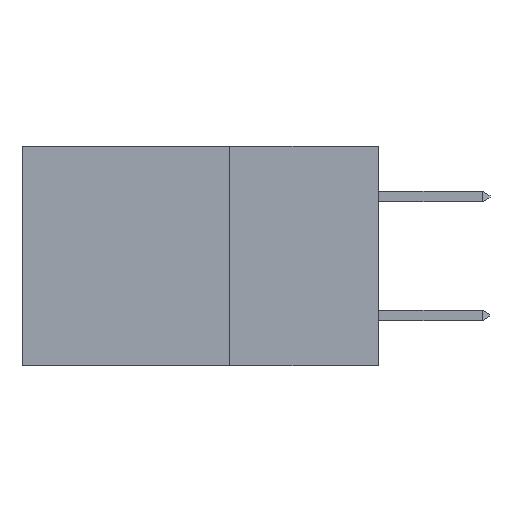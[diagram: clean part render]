
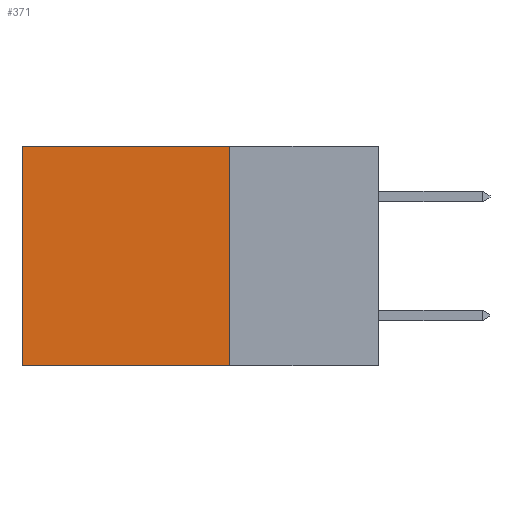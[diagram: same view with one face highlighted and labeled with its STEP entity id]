
A CAD part, left-side view. The second image highlights one B-rep face of the part: STEP entity #371.
In plain terms, the highlighted planar face has unit normal (-1, 0, 0).
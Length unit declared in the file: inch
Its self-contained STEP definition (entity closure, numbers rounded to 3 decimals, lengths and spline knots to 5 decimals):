
#371 = ADVANCED_FACE ( 'NONE', ( #16204 ), #21209, .F. ) ;
#437 = DIRECTION ( 'NONE',  ( 0., 0., -1. ) ) ;
#588 = LINE ( 'NONE', #5844, #9871 ) ;
#594 = DIRECTION ( 'NONE',  ( 1., 0., 0. ) ) ;
#700 = CARTESIAN_POINT ( 'NONE',  ( 0.298, 0.25, 0. ) ) ;
#2138 = CARTESIAN_POINT ( 'NONE',  ( 0.298, 0.25, 0. ) ) ;
#2840 = ORIENTED_EDGE ( 'NONE', *, *, #19943, .T. ) ;
#3973 = DIRECTION ( 'NONE',  ( 0., 1., 0. ) ) ;
#4459 = CARTESIAN_POINT ( 'NONE',  ( 0.298, 0.6, 0. ) ) ;
#4568 = LINE ( 'NONE', #14519, #19767 ) ;
#5844 = CARTESIAN_POINT ( 'NONE',  ( 0.298, 0.25, 0. ) ) ;
#6320 = VECTOR ( 'NONE', #3973, 39.37008 ) ;
#6471 = VERTEX_POINT ( 'NONE', #9774 ) ;
#6593 = CARTESIAN_POINT ( 'NONE',  ( 0.298, 0.6, -0.37 ) ) ;
#6660 = DIRECTION ( 'NONE',  ( 0., 0., -1. ) ) ;
#7316 = CARTESIAN_POINT ( 'NONE',  ( 0.298, 0.25, 0. ) ) ;
#7697 = DIRECTION ( 'NONE',  ( 0., 0., -1. ) ) ;
#8501 = EDGE_CURVE ( 'NONE', #21553, #23458, #11255, .T. ) ;
#8518 = EDGE_LOOP ( 'NONE', ( #2840, #14229, #15672, #9658 ) ) ;
#9658 = ORIENTED_EDGE ( 'NONE', *, *, #8501, .T. ) ;
#9774 = CARTESIAN_POINT ( 'NONE',  ( 0.298, 0.25, -0.37 ) ) ;
#9871 = VECTOR ( 'NONE', #7697, 39.37008 ) ;
#11255 = LINE ( 'NONE', #2138, #6320 ) ;
#13878 = VERTEX_POINT ( 'NONE', #6593 ) ;
#14229 = ORIENTED_EDGE ( 'NONE', *, *, #21485, .F. ) ;
#14519 = CARTESIAN_POINT ( 'NONE',  ( 0.298, 0.25, -0.37 ) ) ;
#15672 = ORIENTED_EDGE ( 'NONE', *, *, #20323, .F. ) ;
#16204 = FACE_OUTER_BOUND ( 'NONE', #8518, .T. ) ;
#17720 = CARTESIAN_POINT ( 'NONE',  ( 0.298, 0.6, 0. ) ) ;
#19767 = VECTOR ( 'NONE', #19860, 39.37008 ) ;
#19860 = DIRECTION ( 'NONE',  ( 0., 1., 0. ) ) ;
#19943 = EDGE_CURVE ( 'NONE', #23458, #13878, #22610, .T. ) ;
#20091 = AXIS2_PLACEMENT_3D ( 'NONE', #700, #594, #437 ) ;
#20323 = EDGE_CURVE ( 'NONE', #21553, #6471, #588, .T. ) ;
#21209 = PLANE ( 'NONE',  #20091 ) ;
#21485 = EDGE_CURVE ( 'NONE', #6471, #13878, #4568, .T. ) ;
#21553 = VERTEX_POINT ( 'NONE', #7316 ) ;
#22610 = LINE ( 'NONE', #17720, #23191 ) ;
#23191 = VECTOR ( 'NONE', #6660, 39.37008 ) ;
#23458 = VERTEX_POINT ( 'NONE', #4459 ) ;
